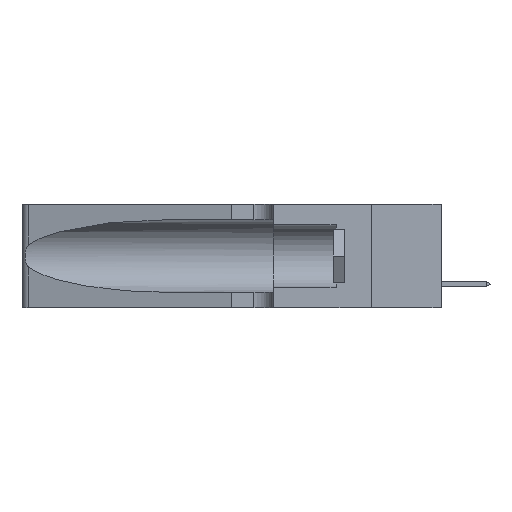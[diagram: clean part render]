
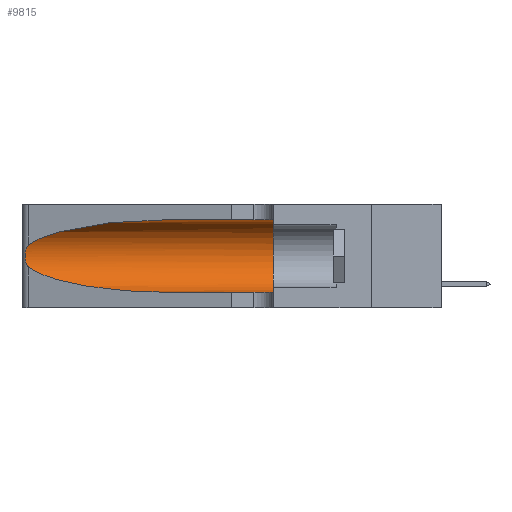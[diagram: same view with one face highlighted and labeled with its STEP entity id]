
A CAD part, left-side view. The second image highlights one B-rep face of the part: STEP entity #9815.
In plain terms, the highlighted cylindrical face has radius 3.308 mm (diameter 6.617 mm), a partial arc.
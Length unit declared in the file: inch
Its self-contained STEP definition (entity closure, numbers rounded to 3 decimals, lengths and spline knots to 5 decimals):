
#112 = DIRECTION ( 'NONE',  ( 0., -1., 0. ) ) ;
#625 = CARTESIAN_POINT ( 'NONE',  ( 0.25487, 1.22718, 0.14631 ) ) ;
#1472 = CARTESIAN_POINT ( 'NONE',  ( 0.25787, 1.23484, 0.2124 ) ) ;
#1750 = EDGE_CURVE ( 'NONE', #13633, #30303, #23288, .T. ) ;
#1979 = CARTESIAN_POINT ( 'NONE',  ( 0.2373, 1.15595, 0.28018 ) ) ;
#2674 = VECTOR ( 'NONE', #112, 39.37008 ) ;
#3365 = CARTESIAN_POINT ( 'NONE',  ( 0.18966, 0.96281, 0.05475 ) ) ;
#3607 = CARTESIAN_POINT ( 'NONE',  ( 0.2373, 1.15595, 0.08982 ) ) ;
#4854 = ORIENTED_EDGE ( 'NONE', *, *, #16743, .T. ) ;
#4920 = CARTESIAN_POINT ( 'NONE',  ( 0.18966, 0.96281, 0.31525 ) ) ;
#5036 = DIRECTION ( 'NONE',  ( 0., 1., 0. ) ) ;
#5719 = DIRECTION ( 'NONE',  ( 0., 0., -1. ) ) ;
#6425 =( BOUNDED_CURVE ( )  B_SPLINE_CURVE ( 3, ( #625, #3607, #3365, #17213 ),
 .UNSPECIFIED., .F., .T. ) 
 B_SPLINE_CURVE_WITH_KNOTS ( ( 4, 4 ),
 ( 3.44316, 4.71239 ),
 .UNSPECIFIED. ) 
 CURVE ( )  GEOMETRIC_REPRESENTATION_ITEM ( )  RATIONAL_B_SPLINE_CURVE ( ( 1., 0.87, 0.87, 1. ) ) 
 REPRESENTATION_ITEM ( '' )  );
#6557 = EDGE_CURVE ( 'NONE', #13633, #35124, #15643, .T. ) ;
#7586 = EDGE_CURVE ( 'NONE', #35124, #12827, #23325, .T. ) ;
#7727 = CARTESIAN_POINT ( 'NONE',  ( 0.25487, 1.22718, 0.22369 ) ) ;
#8294 = DIRECTION ( 'NONE',  ( 0., -1., 0. ) ) ;
#8477 = FACE_OUTER_BOUND ( 'NONE', #11946, .T. ) ;
#9570 = CARTESIAN_POINT ( 'NONE',  ( 0.25789, 1.23486, 0.15765 ) ) ;
#9815 = ADVANCED_FACE ( 'NONE', ( #8477 ), #34794, .F. ) ;
#11762 = CARTESIAN_POINT ( 'NONE',  ( 0.1305, 0.35, 0.05475 ) ) ;
#11946 = EDGE_LOOP ( 'NONE', ( #17820, #30952, #13047, #4854, #15669, #16147 ) ) ;
#12105 = CARTESIAN_POINT ( 'NONE',  ( 0.25639, 1.23184, 0.21858 ) ) ;
#12348 = CARTESIAN_POINT ( 'NONE',  ( 0.25639, 1.23186, 0.15144 ) ) ;
#12476 = CARTESIAN_POINT ( 'NONE',  ( 0.26075, 1.23896, 0.178 ) ) ;
#12482 = CARTESIAN_POINT ( 'NONE',  ( 0.1305, 0.72297, 0.05475 ) ) ;
#12601 = CARTESIAN_POINT ( 'NONE',  ( 0.25854, 1.2359, 0.20912 ) ) ;
#12827 = VERTEX_POINT ( 'NONE', #15368 ) ;
#13047 = ORIENTED_EDGE ( 'NONE', *, *, #32055, .T. ) ;
#13356 = DIRECTION ( 'NONE',  ( 0., 0., 1. ) ) ;
#13633 = VERTEX_POINT ( 'NONE', #33124 ) ;
#14199 = VERTEX_POINT ( 'NONE', #11762 ) ;
#14945 = CARTESIAN_POINT ( 'NONE',  ( 0.26018, 1.23835, 0.19895 ) ) ;
#15368 = CARTESIAN_POINT ( 'NONE',  ( 0.25487, 1.22718, 0.14631 ) ) ;
#15643 =( BOUNDED_CURVE ( )  B_SPLINE_CURVE ( 3, ( #22010, #4920, #1979, #7727 ),
 .UNSPECIFIED., .F., .T. ) 
 B_SPLINE_CURVE_WITH_KNOTS ( ( 4, 4 ),
 ( 1.5708, 2.84003 ),
 .UNSPECIFIED. ) 
 CURVE ( )  GEOMETRIC_REPRESENTATION_ITEM ( )  RATIONAL_B_SPLINE_CURVE ( ( 1., 0.87, 0.87, 1. ) ) 
 REPRESENTATION_ITEM ( '' )  );
#15669 = ORIENTED_EDGE ( 'NONE', *, *, #24947, .F. ) ;
#16147 = ORIENTED_EDGE ( 'NONE', *, *, #1750, .F. ) ;
#16445 = VERTEX_POINT ( 'NONE', #12482 ) ;
#16743 = EDGE_CURVE ( 'NONE', #16445, #14199, #35811, .T. ) ;
#17213 = CARTESIAN_POINT ( 'NONE',  ( 0.1305, 0.72297, 0.05475 ) ) ;
#17390 = DIRECTION ( 'NONE',  ( 0., -1., 0. ) ) ;
#17820 = ORIENTED_EDGE ( 'NONE', *, *, #6557, .T. ) ;
#17918 = CARTESIAN_POINT ( 'NONE',  ( 0.26075, 1.23896, 0.19203 ) ) ;
#18436 = CARTESIAN_POINT ( 'NONE',  ( 0.25487, 1.22718, 0.22369 ) ) ;
#20640 = CARTESIAN_POINT ( 'NONE',  ( 0.26017, 1.23833, 0.17102 ) ) ;
#20887 = VECTOR ( 'NONE', #17390, 39.37008 ) ;
#21018 = CARTESIAN_POINT ( 'NONE',  ( 0.25555, 1.22993, 0.14849 ) ) ;
#22010 = CARTESIAN_POINT ( 'NONE',  ( 0.1305, 0.72297, 0.31525 ) ) ;
#23288 = LINE ( 'NONE', #33742, #2674 ) ;
#23325 = B_SPLINE_CURVE_WITH_KNOTS ( 'NONE', 3,
 ( #29144, #34842, #12105, #1472, #12601, #14945, #17918, #12476, #20640, #35089, #9570, #12348, #21018, #26191 ),
 .UNSPECIFIED., .F., .F.,
 ( 4, 2, 2, 2, 2, 2, 4 ),
 ( 0., 0.00027, 0.00053, 0.00107, 0.0016, 0.00187, 0.00214 ),
 .UNSPECIFIED. ) ;
#24463 = CARTESIAN_POINT ( 'NONE',  ( 0.1305, 0.35, 0.185 ) ) ;
#24766 = CIRCLE ( 'NONE', #25960, 0.13025 ) ;
#24947 = EDGE_CURVE ( 'NONE', #30303, #14199, #24766, .T. ) ;
#25614 = CARTESIAN_POINT ( 'NONE',  ( 0.1305, 1.61858, 0.185 ) ) ;
#25960 = AXIS2_PLACEMENT_3D ( 'NONE', #24463, #5036, #13356 ) ;
#26191 = CARTESIAN_POINT ( 'NONE',  ( 0.25487, 1.22718, 0.14631 ) ) ;
#29144 = CARTESIAN_POINT ( 'NONE',  ( 0.25487, 1.22718, 0.22369 ) ) ;
#30303 = VERTEX_POINT ( 'NONE', #34425 ) ;
#30952 = ORIENTED_EDGE ( 'NONE', *, *, #7586, .T. ) ;
#31782 = CARTESIAN_POINT ( 'NONE',  ( 0.1305, 1.61858, 0.05475 ) ) ;
#32055 = EDGE_CURVE ( 'NONE', #12827, #16445, #6425, .T. ) ;
#33124 = CARTESIAN_POINT ( 'NONE',  ( 0.1305, 0.72297, 0.31525 ) ) ;
#33742 = CARTESIAN_POINT ( 'NONE',  ( 0.1305, 1.61858, 0.31525 ) ) ;
#34425 = CARTESIAN_POINT ( 'NONE',  ( 0.1305, 0.35, 0.31525 ) ) ;
#34794 = CYLINDRICAL_SURFACE ( 'NONE', #35822, 0.13025 ) ;
#34842 = CARTESIAN_POINT ( 'NONE',  ( 0.25555, 1.22994, 0.2215 ) ) ;
#35089 = CARTESIAN_POINT ( 'NONE',  ( 0.25856, 1.23593, 0.16098 ) ) ;
#35124 = VERTEX_POINT ( 'NONE', #18436 ) ;
#35811 = LINE ( 'NONE', #31782, #20887 ) ;
#35822 = AXIS2_PLACEMENT_3D ( 'NONE', #25614, #8294, #5719 ) ;
